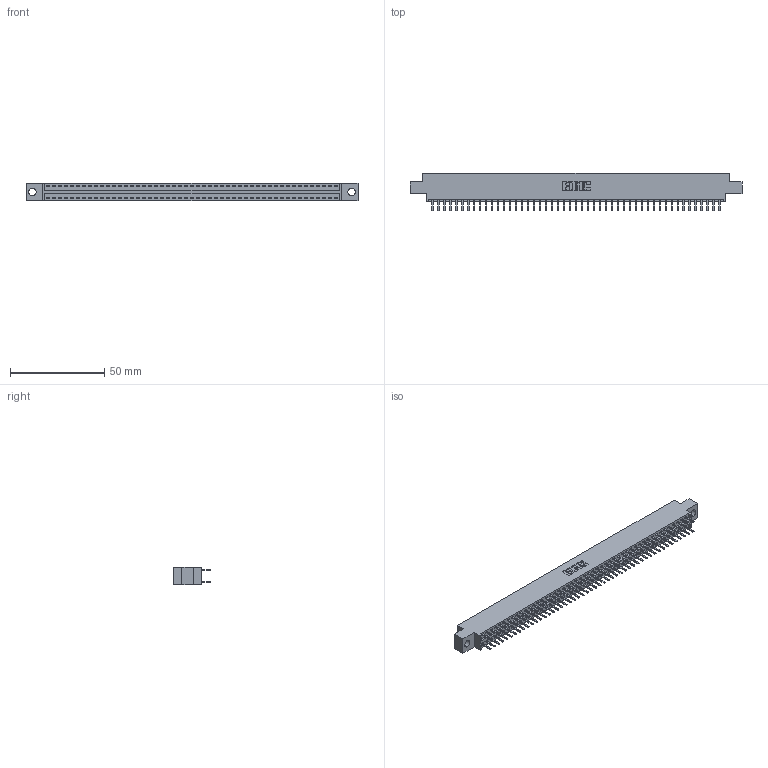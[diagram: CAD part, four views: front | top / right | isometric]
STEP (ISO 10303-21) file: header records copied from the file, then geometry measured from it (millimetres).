
FILE_DESCRIPTION (( 'STEP AP203' ), '1' );
FILE_NAME ('346-098-520-804.STEP', '2022-05-26T17:44:47', ( '' ), ( '' ), 'SwSTEP 2.0', 'SolidWorks 2020', '' );
FILE_SCHEMA (( 'CONFIG_CONTROL_DESIGN' ));
Length unit declared in the file: inch
Products named in the file (3): 345-292-001_345-293-120; 346-098-520-804; 346 Part_0.170 Offset - 0.156 Dia-TH
Assembly tree (99 placements, depth 2):
  346-098-520-804
    346 Part_0.170 Offset - 0.156 Dia-TH
    345-292-001_345-293-120  x98
Bounding box: 176.15 x 20.02 x 9.4 mm (x, y, z)
Volume: 16927.4 mm3; surface area: 23304.5 mm2
Topology: 99 solids, 99 shells, 5628 faces, 16351 edges, 10638 vertices
Faces by surface type: plane 3720, cylinder 1908
Entity records: 31701 total; most frequent: CARTESIAN_POINT 5234, ORIENTED_EDGE 5154, DIRECTION 4649, EDGE_CURVE 2577, LINE 2245, VECTOR 2245, VERTEX_POINT 1714, AXIS2_PLACEMENT_3D 1202
